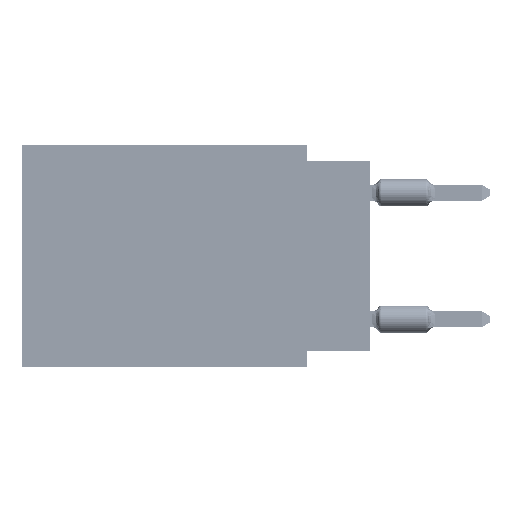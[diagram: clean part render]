
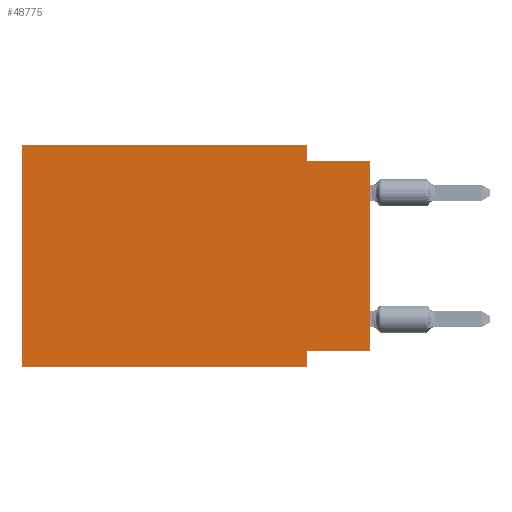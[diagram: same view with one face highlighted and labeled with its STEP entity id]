
A CAD part, left-side view. The second image highlights one B-rep face of the part: STEP entity #48775.
In plain terms, the highlighted planar face has unit normal (-1, 0, 0).
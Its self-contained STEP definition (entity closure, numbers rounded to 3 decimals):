
#1994 = EDGE_LOOP ( 'NONE', ( #40159, #10252, #21968, #38448, #54876, #98546, #58731, #90399 ) ) ;
#6420 = VERTEX_POINT ( 'NONE', #60314 ) ;
#6783 = VECTOR ( 'NONE', #15787, 1000. ) ;
#6853 = EDGE_CURVE ( 'NONE', #66819, #10971, #30937, .T. ) ;
#8775 = EDGE_CURVE ( 'NONE', #91119, #63390, #36989, .T. ) ;
#10252 = ORIENTED_EDGE ( 'NONE', *, *, #23378, .F. ) ;
#10971 = VERTEX_POINT ( 'NONE', #44074 ) ;
#11385 = VERTEX_POINT ( 'NONE', #54240 ) ;
#12148 = PLANE ( 'NONE',  #27939 ) ;
#13545 = DIRECTION ( 'NONE',  ( 0., 1., 0. ) ) ;
#13631 = DIRECTION ( 'NONE',  ( 0., -1., 0. ) ) ;
#15514 = VECTOR ( 'NONE', #21924, 1000. ) ;
#15787 = DIRECTION ( 'NONE',  ( 0., 0., -1. ) ) ;
#18371 = LINE ( 'NONE', #59063, #71023 ) ;
#20420 = LINE ( 'NONE', #84597, #89345 ) ;
#20793 = DIRECTION ( 'NONE',  ( 0., 0., -1. ) ) ;
#21448 = CARTESIAN_POINT ( 'NONE',  ( 0., 2.54, -8.255 ) ) ;
#21924 = DIRECTION ( 'NONE',  ( 0., -1., 0. ) ) ;
#21968 = ORIENTED_EDGE ( 'NONE', *, *, #67195, .F. ) ;
#22487 = CARTESIAN_POINT ( 'NONE',  ( 0., 13.97, -8.89 ) ) ;
#22957 = VECTOR ( 'NONE', #20793, 1000. ) ;
#23112 = CARTESIAN_POINT ( 'NONE',  ( 0., 2.54, -8.89 ) ) ;
#23378 = EDGE_CURVE ( 'NONE', #74684, #6420, #85059, .T. ) ;
#27939 = AXIS2_PLACEMENT_3D ( 'NONE', #59669, #83144, #29359 ) ;
#28436 = CARTESIAN_POINT ( 'NONE',  ( 0., 2.54, 0. ) ) ;
#29159 = DIRECTION ( 'NONE',  ( 0., -1., 0. ) ) ;
#29359 = DIRECTION ( 'NONE',  ( 0., 0., -1. ) ) ;
#30937 = LINE ( 'NONE', #23112, #6783 ) ;
#33172 = EDGE_CURVE ( 'NONE', #93639, #10971, #86148, .T. ) ;
#36989 = LINE ( 'NONE', #77670, #95363 ) ;
#37471 = CARTESIAN_POINT ( 'NONE',  ( 0., 2.54, 0. ) ) ;
#37565 = CARTESIAN_POINT ( 'NONE',  ( 0., 13.97, 0. ) ) ;
#37567 = CARTESIAN_POINT ( 'NONE',  ( 0., 0., -0.635 ) ) ;
#38448 = ORIENTED_EDGE ( 'NONE', *, *, #8775, .F. ) ;
#40159 = ORIENTED_EDGE ( 'NONE', *, *, #60732, .T. ) ;
#44074 = CARTESIAN_POINT ( 'NONE',  ( 0., 2.54, -8.89 ) ) ;
#46256 = EDGE_CURVE ( 'NONE', #11385, #66819, #77705, .T. ) ;
#48775 = ADVANCED_FACE ( 'NONE', ( #84163 ), #12148, .F. ) ;
#50195 = DIRECTION ( 'NONE',  ( 0., 0., 1. ) ) ;
#54240 = CARTESIAN_POINT ( 'NONE',  ( 0., 0., -8.255 ) ) ;
#54876 = ORIENTED_EDGE ( 'NONE', *, *, #98471, .F. ) ;
#58731 = ORIENTED_EDGE ( 'NONE', *, *, #6853, .F. ) ;
#59063 = CARTESIAN_POINT ( 'NONE',  ( 0., 0., 0. ) ) ;
#59440 = LINE ( 'NONE', #37471, #22957 ) ;
#59669 = CARTESIAN_POINT ( 'NONE',  ( 0., 13.97, 0. ) ) ;
#60314 = CARTESIAN_POINT ( 'NONE',  ( 0., 0., -0.635 ) ) ;
#60732 = EDGE_CURVE ( 'NONE', #11385, #6420, #18371, .T. ) ;
#61544 = CARTESIAN_POINT ( 'NONE',  ( 0., 0., -8.255 ) ) ;
#61883 = CARTESIAN_POINT ( 'NONE',  ( 0., 2.54, -0.635 ) ) ;
#63390 = VERTEX_POINT ( 'NONE', #28436 ) ;
#66819 = VERTEX_POINT ( 'NONE', #21448 ) ;
#67195 = EDGE_CURVE ( 'NONE', #63390, #74684, #59440, .T. ) ;
#67997 = CARTESIAN_POINT ( 'NONE',  ( 0., 13.97, -8.89 ) ) ;
#71023 = VECTOR ( 'NONE', #50195, 1000. ) ;
#74684 = VERTEX_POINT ( 'NONE', #61883 ) ;
#76240 = DIRECTION ( 'NONE',  ( 0., 0., 1. ) ) ;
#77670 = CARTESIAN_POINT ( 'NONE',  ( 0., 13.97, 0. ) ) ;
#77705 = LINE ( 'NONE', #61544, #89945 ) ;
#83144 = DIRECTION ( 'NONE',  ( 1., 0., 0. ) ) ;
#84163 = FACE_OUTER_BOUND ( 'NONE', #1994, .T. ) ;
#84597 = CARTESIAN_POINT ( 'NONE',  ( 0., 13.97, 0. ) ) ;
#85059 = LINE ( 'NONE', #37567, #15514 ) ;
#86148 = LINE ( 'NONE', #22487, #88328 ) ;
#88328 = VECTOR ( 'NONE', #13631, 1000. ) ;
#89345 = VECTOR ( 'NONE', #76240, 1000. ) ;
#89945 = VECTOR ( 'NONE', #13545, 1000. ) ;
#90399 = ORIENTED_EDGE ( 'NONE', *, *, #46256, .F. ) ;
#91119 = VERTEX_POINT ( 'NONE', #37565 ) ;
#93639 = VERTEX_POINT ( 'NONE', #67997 ) ;
#95363 = VECTOR ( 'NONE', #29159, 1000. ) ;
#98471 = EDGE_CURVE ( 'NONE', #93639, #91119, #20420, .T. ) ;
#98546 = ORIENTED_EDGE ( 'NONE', *, *, #33172, .T. ) ;
